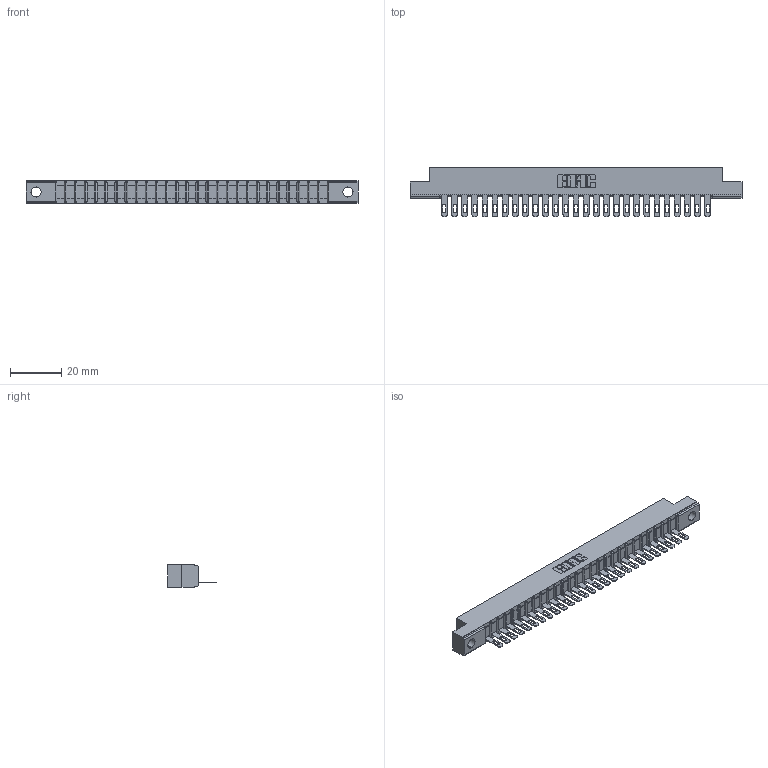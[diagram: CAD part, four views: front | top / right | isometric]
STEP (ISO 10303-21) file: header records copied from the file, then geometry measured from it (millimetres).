
FILE_DESCRIPTION (( 'STEP AP203' ), '1' );
FILE_NAME ('357-027-505-104.STEP', '2019-09-14T02:15:50', ( '' ), ( '' ), 'SwSTEP 2.0', 'SolidWorks 2016', '' );
FILE_SCHEMA (( 'CONFIG_CONTROL_DESIGN' ));
Length unit declared in the file: inch
Products named in the file (3): 357-027-505-104; 307-290-001_505; 307 Part_.156 Dia Mounting Holes
Assembly tree (28 placements, depth 2):
  357-027-505-104
    307 Part_.156 Dia Mounting Holes
    307-290-001_505  x27
Bounding box: 130 x 19.18 x 8.71 mm (x, y, z)
Volume: 8125.7 mm3; surface area: 12874 mm2
Topology: 28 solids, 28 shells, 1672 faces, 4733 edges, 3042 vertices
Faces by surface type: plane 1056, cylinder 560, sphere 56
Entity records: 25388 total; most frequent: CARTESIAN_POINT 4274, ORIENTED_EDGE 4258, DIRECTION 4159, EDGE_CURVE 2129, VECTOR 1633, LINE 1633, VERTEX_POINT 1378, AXIS2_PLACEMENT_3D 1263
